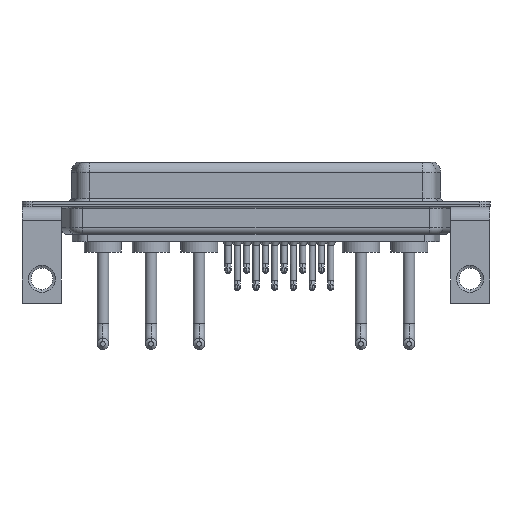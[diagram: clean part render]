
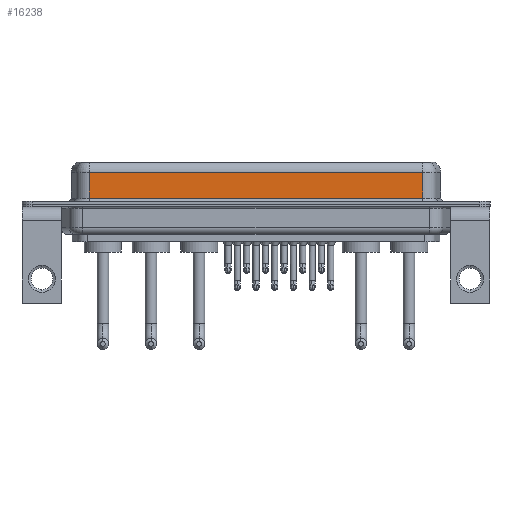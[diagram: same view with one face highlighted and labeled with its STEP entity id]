
A CAD part, front view. The second image highlights one B-rep face of the part: STEP entity #16238.
In plain terms, the highlighted planar face has unit normal (0, -1, 0).
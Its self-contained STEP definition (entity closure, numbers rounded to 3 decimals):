
#156 = EDGE_CURVE ( 'NONE', #10318, #3667, #17235, .T. ) ;
#1844 = CARTESIAN_POINT ( 'NONE',  ( 56.462, -3.95, 4.65 ) ) ;
#2182 = CARTESIAN_POINT ( 'NONE',  ( 56.462, -3.95, 6.4 ) ) ;
#2301 = ORIENTED_EDGE ( 'NONE', *, *, #8468, .T. ) ;
#3484 = EDGE_CURVE ( 'NONE', #13475, #10318, #14856, .T. ) ;
#3662 = PLANE ( 'NONE',  #15412 ) ;
#3667 = VERTEX_POINT ( 'NONE', #19286 ) ;
#3758 = FACE_OUTER_BOUND ( 'NONE', #20290, .T. ) ;
#4085 = DIRECTION ( 'NONE',  ( 0., 0., 1. ) ) ;
#4401 = CARTESIAN_POINT ( 'NONE',  ( 7.038, -3.95, 0.9 ) ) ;
#4696 = VECTOR ( 'NONE', #12657, 1000. ) ;
#5921 = ORIENTED_EDGE ( 'NONE', *, *, #156, .T. ) ;
#6063 = CARTESIAN_POINT ( 'NONE',  ( 56.462, -3.95, 6.4 ) ) ;
#7549 = EDGE_CURVE ( 'NONE', #15017, #3667, #20626, .T. ) ;
#7667 = DIRECTION ( 'NONE',  ( 1., 0., 0. ) ) ;
#7900 = ORIENTED_EDGE ( 'NONE', *, *, #7549, .F. ) ;
#8468 = EDGE_CURVE ( 'NONE', #15017, #13475, #11209, .T. ) ;
#10318 = VERTEX_POINT ( 'NONE', #4401 ) ;
#10894 = VECTOR ( 'NONE', #7667, 1000. ) ;
#11116 = DIRECTION ( 'NONE',  ( -1., 0., 0. ) ) ;
#11209 = LINE ( 'NONE', #17596, #13921 ) ;
#11926 = DIRECTION ( 'NONE',  ( 0., 1., 0. ) ) ;
#12657 = DIRECTION ( 'NONE',  ( 0., 0., -1. ) ) ;
#13475 = VERTEX_POINT ( 'NONE', #14767 ) ;
#13921 = VECTOR ( 'NONE', #11116, 1000. ) ;
#14557 = ORIENTED_EDGE ( 'NONE', *, *, #3484, .T. ) ;
#14767 = CARTESIAN_POINT ( 'NONE',  ( 7.038, -3.95, 4.65 ) ) ;
#14856 = LINE ( 'NONE', #16442, #19783 ) ;
#15017 = VERTEX_POINT ( 'NONE', #1844 ) ;
#15412 = AXIS2_PLACEMENT_3D ( 'NONE', #2182, #11926, #4085 ) ;
#16238 = ADVANCED_FACE ( 'NONE', ( #3758 ), #3662, .F. ) ;
#16442 = CARTESIAN_POINT ( 'NONE',  ( 7.038, -3.95, 6.4 ) ) ;
#16546 = DIRECTION ( 'NONE',  ( 0., 0., -1. ) ) ;
#17235 = LINE ( 'NONE', #19153, #10894 ) ;
#17596 = CARTESIAN_POINT ( 'NONE',  ( 56.462, -3.95, 4.65 ) ) ;
#19153 = CARTESIAN_POINT ( 'NONE',  ( 56.462, -3.95, 0.9 ) ) ;
#19286 = CARTESIAN_POINT ( 'NONE',  ( 56.462, -3.95, 0.9 ) ) ;
#19783 = VECTOR ( 'NONE', #16546, 1000. ) ;
#20290 = EDGE_LOOP ( 'NONE', ( #7900, #2301, #14557, #5921 ) ) ;
#20626 = LINE ( 'NONE', #6063, #4696 ) ;
